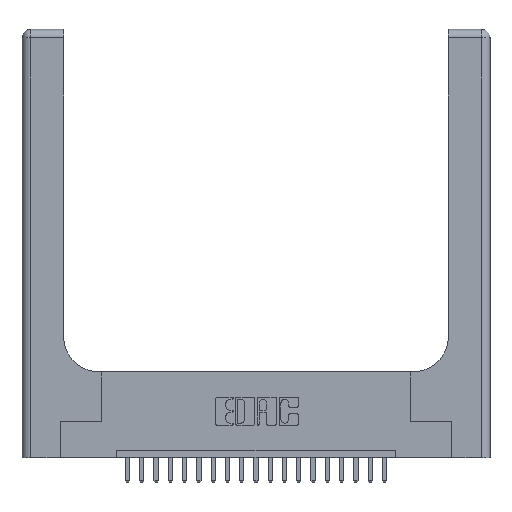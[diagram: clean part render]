
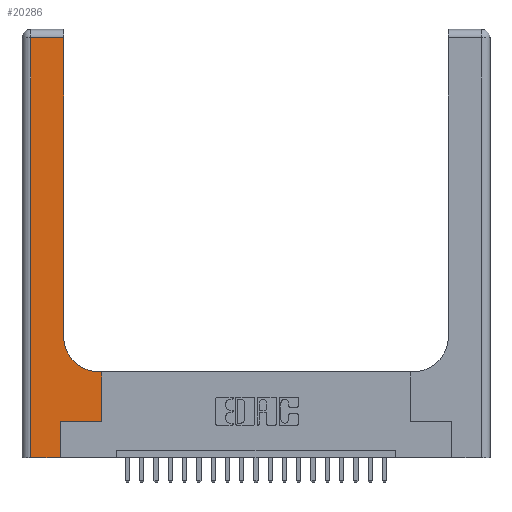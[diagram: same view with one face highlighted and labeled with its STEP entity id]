
A CAD part, top view. The second image highlights one B-rep face of the part: STEP entity #20286.
In plain terms, the highlighted planar face has unit normal (0, 0, 1).
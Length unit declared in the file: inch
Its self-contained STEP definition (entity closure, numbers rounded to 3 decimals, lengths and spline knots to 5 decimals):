
#107 = DIRECTION ( 'NONE',  ( -1., 0., 0. ) ) ;
#231 = EDGE_CURVE ( 'NONE', #16317, #3538, #18304, .T. ) ;
#320 = VECTOR ( 'NONE', #4129, 39.37008 ) ;
#383 = CARTESIAN_POINT ( 'NONE',  ( 0.2915, 3., 0.37 ) ) ;
#423 = CARTESIAN_POINT ( 'NONE',  ( 0.5585, 0.25, 0.37 ) ) ;
#537 = ORIENTED_EDGE ( 'NONE', *, *, #3476, .T. ) ;
#636 = LINE ( 'NONE', #2451, #17697 ) ;
#1077 = VERTEX_POINT ( 'NONE', #6118 ) ;
#1318 = DIRECTION ( 'NONE',  ( 1., 0., 0. ) ) ;
#1839 = AXIS2_PLACEMENT_3D ( 'NONE', #2158, #21307, #107 ) ;
#2065 = DIRECTION ( 'NONE',  ( 0., 1., 0. ) ) ;
#2158 = CARTESIAN_POINT ( 'NONE',  ( 0., 3., 0.37 ) ) ;
#2451 = CARTESIAN_POINT ( 'NONE',  ( 0., 2.94, 0.37 ) ) ;
#2950 = ORIENTED_EDGE ( 'NONE', *, *, #231, .T. ) ;
#3054 = EDGE_LOOP ( 'NONE', ( #15954, #16735, #17819, #11390, #10894, #2950, #537, #4489, #3070 ) ) ;
#3070 = ORIENTED_EDGE ( 'NONE', *, *, #7380, .T. ) ;
#3476 = EDGE_CURVE ( 'NONE', #3538, #1077, #7188, .T. ) ;
#3538 = VERTEX_POINT ( 'NONE', #7856 ) ;
#3837 = DIRECTION ( 'NONE',  ( 0., 1., 0. ) ) ;
#4090 = CARTESIAN_POINT ( 'NONE',  ( 0.269, 0., 0.37 ) ) ;
#4129 = DIRECTION ( 'NONE',  ( 1., 0., 0. ) ) ;
#4246 = VERTEX_POINT ( 'NONE', #15602 ) ;
#4489 = ORIENTED_EDGE ( 'NONE', *, *, #5006, .T. ) ;
#4518 = LINE ( 'NONE', #19235, #320 ) ;
#4613 = VECTOR ( 'NONE', #1318, 39.37008 ) ;
#5006 = EDGE_CURVE ( 'NONE', #1077, #8853, #8215, .T. ) ;
#5335 = VERTEX_POINT ( 'NONE', #21699 ) ;
#5505 = PLANE ( 'NONE',  #1839 ) ;
#5660 = VECTOR ( 'NONE', #2065, 39.37008 ) ;
#6118 = CARTESIAN_POINT ( 'NONE',  ( 0.5585, 0.6, 0.37 ) ) ;
#6382 = CARTESIAN_POINT ( 'NONE',  ( 0.269, 0.25, 0.37 ) ) ;
#6400 = EDGE_CURVE ( 'NONE', #18751, #16317, #16094, .T. ) ;
#6935 = DIRECTION ( 'NONE',  ( 0., -1., 0. ) ) ;
#7188 = LINE ( 'NONE', #423, #17293 ) ;
#7254 = CIRCLE ( 'NONE', #8844, 0.25 ) ;
#7380 = EDGE_CURVE ( 'NONE', #8853, #5335, #7254, .T. ) ;
#7856 = CARTESIAN_POINT ( 'NONE',  ( 0.5585, 0.25, 0.37 ) ) ;
#8211 = VERTEX_POINT ( 'NONE', #19083 ) ;
#8215 = LINE ( 'NONE', #12274, #10939 ) ;
#8323 = LINE ( 'NONE', #383, #18748 ) ;
#8844 = AXIS2_PLACEMENT_3D ( 'NONE', #17540, #16073, #14223 ) ;
#8853 = VERTEX_POINT ( 'NONE', #17010 ) ;
#10491 = VECTOR ( 'NONE', #6935, 39.37008 ) ;
#10853 = VERTEX_POINT ( 'NONE', #21589 ) ;
#10894 = ORIENTED_EDGE ( 'NONE', *, *, #6400, .T. ) ;
#10939 = VECTOR ( 'NONE', #15634, 39.37008 ) ;
#11390 = ORIENTED_EDGE ( 'NONE', *, *, #17100, .T. ) ;
#11391 = DIRECTION ( 'NONE',  ( -1., 0., 0. ) ) ;
#12094 = CARTESIAN_POINT ( 'NONE',  ( 0.269, 0.25, 0.37 ) ) ;
#12274 = CARTESIAN_POINT ( 'NONE',  ( 0.2915, 0.6, 0.37 ) ) ;
#12940 = DIRECTION ( 'NONE',  ( 0., 1., 0. ) ) ;
#13722 = FACE_OUTER_BOUND ( 'NONE', #3054, .T. ) ;
#14223 = DIRECTION ( 'NONE',  ( 1., 0., 0. ) ) ;
#14268 = EDGE_CURVE ( 'NONE', #8211, #4246, #636, .T. ) ;
#14565 = CARTESIAN_POINT ( 'NONE',  ( 0.269, 0., 0.37 ) ) ;
#15602 = CARTESIAN_POINT ( 'NONE',  ( 0.06, 2.94, 0.37 ) ) ;
#15634 = DIRECTION ( 'NONE',  ( -1., 0., 0. ) ) ;
#15954 = ORIENTED_EDGE ( 'NONE', *, *, #18269, .T. ) ;
#16073 = DIRECTION ( 'NONE',  ( 0., 0., -1. ) ) ;
#16094 = LINE ( 'NONE', #4090, #5660 ) ;
#16234 = LINE ( 'NONE', #19260, #10491 ) ;
#16269 = EDGE_CURVE ( 'NONE', #4246, #10853, #16234, .T. ) ;
#16317 = VERTEX_POINT ( 'NONE', #6382 ) ;
#16735 = ORIENTED_EDGE ( 'NONE', *, *, #14268, .T. ) ;
#17010 = CARTESIAN_POINT ( 'NONE',  ( 0.5415, 0.6, 0.37 ) ) ;
#17100 = EDGE_CURVE ( 'NONE', #10853, #18751, #4518, .T. ) ;
#17293 = VECTOR ( 'NONE', #3837, 39.37008 ) ;
#17540 = CARTESIAN_POINT ( 'NONE',  ( 0.5415, 0.85, 0.37 ) ) ;
#17697 = VECTOR ( 'NONE', #11391, 39.37008 ) ;
#17819 = ORIENTED_EDGE ( 'NONE', *, *, #16269, .T. ) ;
#18269 = EDGE_CURVE ( 'NONE', #5335, #8211, #8323, .T. ) ;
#18304 = LINE ( 'NONE', #12094, #4613 ) ;
#18748 = VECTOR ( 'NONE', #12940, 39.37008 ) ;
#18751 = VERTEX_POINT ( 'NONE', #14565 ) ;
#19083 = CARTESIAN_POINT ( 'NONE',  ( 0.2915, 2.94, 0.37 ) ) ;
#19235 = CARTESIAN_POINT ( 'NONE',  ( 0., 0., 0.37 ) ) ;
#19260 = CARTESIAN_POINT ( 'NONE',  ( 0.06, 3., 0.37 ) ) ;
#20286 = ADVANCED_FACE ( 'NONE', ( #13722 ), #5505, .F. ) ;
#21307 = DIRECTION ( 'NONE',  ( 0., 0., -1. ) ) ;
#21589 = CARTESIAN_POINT ( 'NONE',  ( 0.06, 0., 0.37 ) ) ;
#21699 = CARTESIAN_POINT ( 'NONE',  ( 0.2915, 0.85, 0.37 ) ) ;
